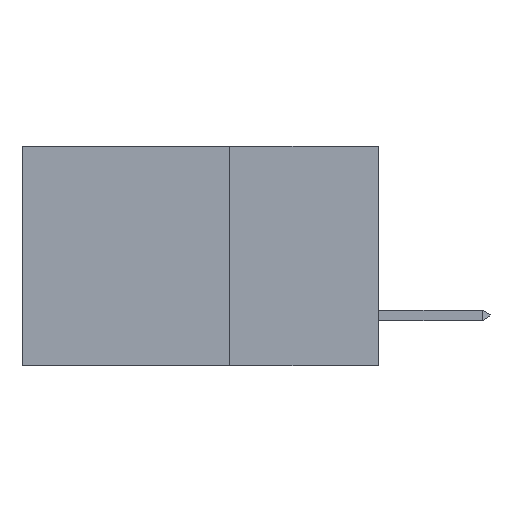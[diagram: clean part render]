
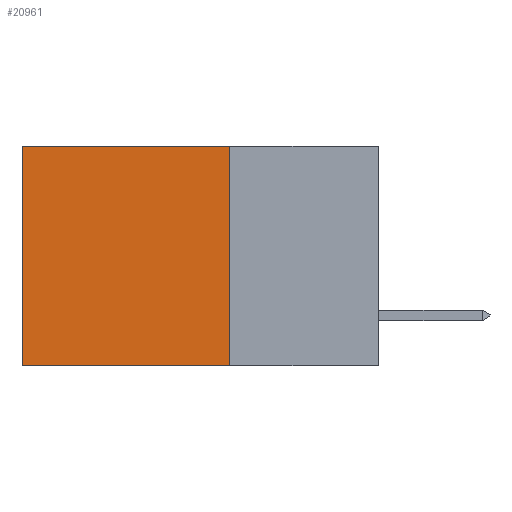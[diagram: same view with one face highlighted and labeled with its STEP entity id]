
A CAD part, left-side view. The second image highlights one B-rep face of the part: STEP entity #20961.
In plain terms, the highlighted planar face has unit normal (-1, 0, 0).
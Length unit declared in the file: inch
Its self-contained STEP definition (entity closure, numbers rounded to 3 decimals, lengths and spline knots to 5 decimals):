
#373 = VECTOR ( 'NONE', #8250, 39.37008 ) ;
#1736 = CARTESIAN_POINT ( 'NONE',  ( 0.298, 0.6, -0.37 ) ) ;
#2678 = ORIENTED_EDGE ( 'NONE', *, *, #18077, .T. ) ;
#5008 = DIRECTION ( 'NONE',  ( 1., 0., 0. ) ) ;
#5019 = CARTESIAN_POINT ( 'NONE',  ( 0.298, 0.25, 0. ) ) ;
#5585 = LINE ( 'NONE', #19199, #8925 ) ;
#7550 = VERTEX_POINT ( 'NONE', #5019 ) ;
#8250 = DIRECTION ( 'NONE',  ( 0., 1., 0. ) ) ;
#8322 = DIRECTION ( 'NONE',  ( 0., 0., -1. ) ) ;
#8925 = VECTOR ( 'NONE', #16900, 39.37008 ) ;
#9183 = VECTOR ( 'NONE', #21892, 39.37008 ) ;
#9861 = CARTESIAN_POINT ( 'NONE',  ( 0.298, 0.25, -0.37 ) ) ;
#10512 = VERTEX_POINT ( 'NONE', #1736 ) ;
#10768 = PLANE ( 'NONE',  #21153 ) ;
#11645 = EDGE_CURVE ( 'NONE', #18122, #10512, #24085, .T. ) ;
#12661 = FACE_OUTER_BOUND ( 'NONE', #24908, .T. ) ;
#15479 = ORIENTED_EDGE ( 'NONE', *, *, #24873, .F. ) ;
#15933 = CARTESIAN_POINT ( 'NONE',  ( 0.298, 0.25, -0.37 ) ) ;
#16562 = LINE ( 'NONE', #17836, #22652 ) ;
#16896 = EDGE_CURVE ( 'NONE', #20619, #10512, #5585, .T. ) ;
#16900 = DIRECTION ( 'NONE',  ( 0., 0., -1. ) ) ;
#17819 = CARTESIAN_POINT ( 'NONE',  ( 0.298, 0.25, 0. ) ) ;
#17836 = CARTESIAN_POINT ( 'NONE',  ( 0.298, 0.25, 0. ) ) ;
#18077 = EDGE_CURVE ( 'NONE', #7550, #20619, #20080, .T. ) ;
#18122 = VERTEX_POINT ( 'NONE', #15933 ) ;
#19199 = CARTESIAN_POINT ( 'NONE',  ( 0.298, 0.6, 0. ) ) ;
#20080 = LINE ( 'NONE', #17819, #9183 ) ;
#20619 = VERTEX_POINT ( 'NONE', #24198 ) ;
#20961 = ADVANCED_FACE ( 'NONE', ( #12661 ), #10768, .F. ) ;
#21058 = ORIENTED_EDGE ( 'NONE', *, *, #11645, .F. ) ;
#21153 = AXIS2_PLACEMENT_3D ( 'NONE', #22720, #5008, #24330 ) ;
#21892 = DIRECTION ( 'NONE',  ( 0., 1., 0. ) ) ;
#22652 = VECTOR ( 'NONE', #8322, 39.37008 ) ;
#22720 = CARTESIAN_POINT ( 'NONE',  ( 0.298, 0.25, 0. ) ) ;
#22888 = ORIENTED_EDGE ( 'NONE', *, *, #16896, .T. ) ;
#24085 = LINE ( 'NONE', #9861, #373 ) ;
#24198 = CARTESIAN_POINT ( 'NONE',  ( 0.298, 0.6, 0. ) ) ;
#24330 = DIRECTION ( 'NONE',  ( 0., 0., -1. ) ) ;
#24873 = EDGE_CURVE ( 'NONE', #7550, #18122, #16562, .T. ) ;
#24908 = EDGE_LOOP ( 'NONE', ( #22888, #21058, #15479, #2678 ) ) ;
